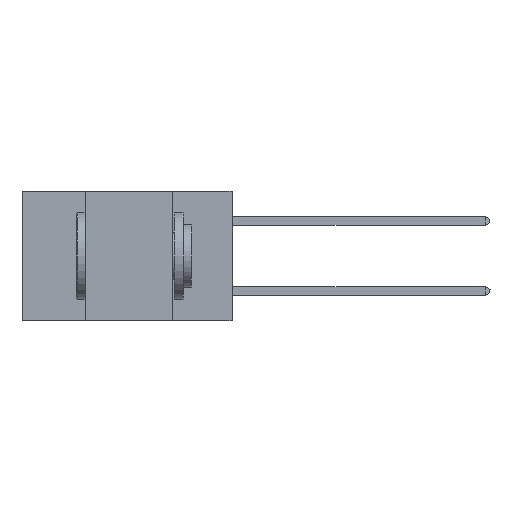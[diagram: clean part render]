
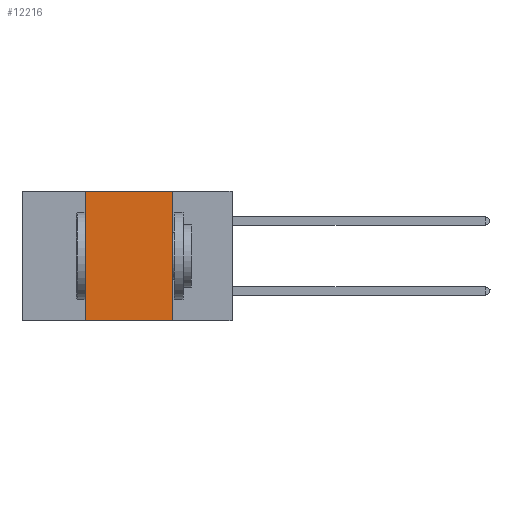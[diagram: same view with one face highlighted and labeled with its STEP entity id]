
A CAD part, left-side view. The second image highlights one B-rep face of the part: STEP entity #12216.
In plain terms, the highlighted planar face has unit normal (-1, 0, 0).
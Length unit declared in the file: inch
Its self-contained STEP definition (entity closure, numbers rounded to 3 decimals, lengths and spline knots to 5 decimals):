
#401 = VERTEX_POINT ( 'NONE', #23119 ) ;
#2488 = EDGE_CURVE ( 'NONE', #13325, #3953, #7529, .T. ) ;
#3262 = VERTEX_POINT ( 'NONE', #22523 ) ;
#3739 = DIRECTION ( 'NONE',  ( 0., -1., 0. ) ) ;
#3953 = VERTEX_POINT ( 'NONE', #16614 ) ;
#5002 = CARTESIAN_POINT ( 'NONE',  ( 0., 0.6, 0. ) ) ;
#6521 = DIRECTION ( 'NONE',  ( 0., 0., 1. ) ) ;
#6843 = VECTOR ( 'NONE', #3739, 39.37008 ) ;
#6916 = AXIS2_PLACEMENT_3D ( 'NONE', #5002, #22248, #9346 ) ;
#7525 = ORIENTED_EDGE ( 'NONE', *, *, #2488, .T. ) ;
#7529 = LINE ( 'NONE', #16670, #6843 ) ;
#8031 = VECTOR ( 'NONE', #6521, 39.37008 ) ;
#8799 = ORIENTED_EDGE ( 'NONE', *, *, #15730, .F. ) ;
#9346 = DIRECTION ( 'NONE',  ( 0., 0., -1. ) ) ;
#9454 = CARTESIAN_POINT ( 'NONE',  ( 0., 0.6, 0. ) ) ;
#12216 = ADVANCED_FACE ( 'NONE', ( #14111 ), #13948, .F. ) ;
#12485 = EDGE_CURVE ( 'NONE', #13325, #3262, #25182, .T. ) ;
#12970 = CARTESIAN_POINT ( 'NONE',  ( 0., 0.42, 0. ) ) ;
#13325 = VERTEX_POINT ( 'NONE', #15576 ) ;
#13571 = ORIENTED_EDGE ( 'NONE', *, *, #12485, .F. ) ;
#13948 = PLANE ( 'NONE',  #6916 ) ;
#14111 = FACE_OUTER_BOUND ( 'NONE', #27086, .T. ) ;
#15272 = LINE ( 'NONE', #9454, #21348 ) ;
#15576 = CARTESIAN_POINT ( 'NONE',  ( 0., 0.42, -0.37 ) ) ;
#15730 = EDGE_CURVE ( 'NONE', #3262, #401, #15272, .T. ) ;
#16614 = CARTESIAN_POINT ( 'NONE',  ( 0., 0.17, -0.37 ) ) ;
#16670 = CARTESIAN_POINT ( 'NONE',  ( 0., 0.6, -0.37 ) ) ;
#19421 = EDGE_CURVE ( 'NONE', #401, #3953, #22766, .T. ) ;
#20827 = CARTESIAN_POINT ( 'NONE',  ( 0., 0.17, 0. ) ) ;
#21187 = ORIENTED_EDGE ( 'NONE', *, *, #19421, .F. ) ;
#21348 = VECTOR ( 'NONE', #24653, 39.37008 ) ;
#21431 = VECTOR ( 'NONE', #27603, 39.37008 ) ;
#22248 = DIRECTION ( 'NONE',  ( 1., 0., 0. ) ) ;
#22523 = CARTESIAN_POINT ( 'NONE',  ( 0., 0.42, 0. ) ) ;
#22766 = LINE ( 'NONE', #20827, #21431 ) ;
#23119 = CARTESIAN_POINT ( 'NONE',  ( 0., 0.17, 0. ) ) ;
#24653 = DIRECTION ( 'NONE',  ( 0., -1., 0. ) ) ;
#25182 = LINE ( 'NONE', #12970, #8031 ) ;
#27086 = EDGE_LOOP ( 'NONE', ( #21187, #8799, #13571, #7525 ) ) ;
#27603 = DIRECTION ( 'NONE',  ( 0., 0., -1. ) ) ;
